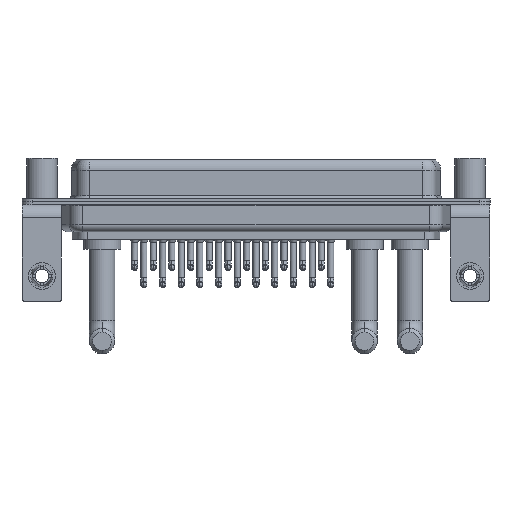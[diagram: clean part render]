
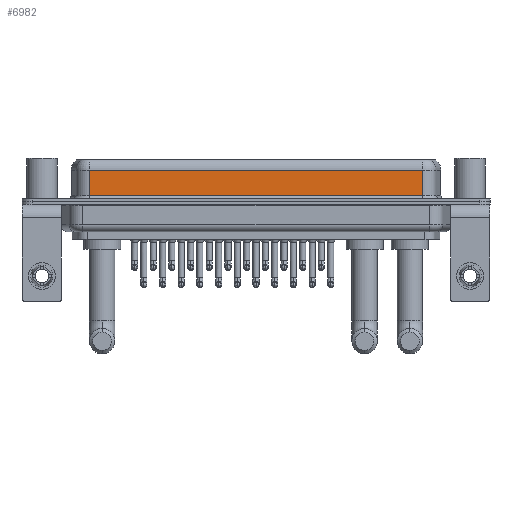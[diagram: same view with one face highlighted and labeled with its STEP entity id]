
A CAD part, front view. The second image highlights one B-rep face of the part: STEP entity #6982.
In plain terms, the highlighted planar face has unit normal (0, -1, 0).
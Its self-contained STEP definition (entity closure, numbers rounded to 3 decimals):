
#1175 = DIRECTION ( 'NONE',  ( 1., 0., 0. ) ) ;
#1801 = CARTESIAN_POINT ( 'NONE',  ( 56.462, -3.95, 6.4 ) ) ;
#2533 = ORIENTED_EDGE ( 'NONE', *, *, #26857, .T. ) ;
#2872 = VECTOR ( 'NONE', #3121, 1000. ) ;
#3121 = DIRECTION ( 'NONE',  ( -1., 0., 0. ) ) ;
#4502 = CARTESIAN_POINT ( 'NONE',  ( 7.038, -3.95, 4.65 ) ) ;
#6108 = DIRECTION ( 'NONE',  ( 0., 0., -1. ) ) ;
#6982 = ADVANCED_FACE ( 'NONE', ( #18783 ), #10620, .F. ) ;
#7758 = ORIENTED_EDGE ( 'NONE', *, *, #14734, .T. ) ;
#7822 = LINE ( 'NONE', #22518, #14104 ) ;
#8000 = CARTESIAN_POINT ( 'NONE',  ( 56.462, -3.95, 6.4 ) ) ;
#8579 = DIRECTION ( 'NONE',  ( 0., 0., -1. ) ) ;
#9319 = CARTESIAN_POINT ( 'NONE',  ( 7.038, -3.95, 0.9 ) ) ;
#9834 = EDGE_CURVE ( 'NONE', #12134, #17858, #7822, .T. ) ;
#10620 = PLANE ( 'NONE',  #21606 ) ;
#12134 = VERTEX_POINT ( 'NONE', #9319 ) ;
#12714 = ORIENTED_EDGE ( 'NONE', *, *, #9834, .T. ) ;
#13174 = CARTESIAN_POINT ( 'NONE',  ( 56.462, -3.95, 4.65 ) ) ;
#13313 = CARTESIAN_POINT ( 'NONE',  ( 56.462, -3.95, 0.9 ) ) ;
#13820 = ORIENTED_EDGE ( 'NONE', *, *, #13949, .F. ) ;
#13949 = EDGE_CURVE ( 'NONE', #15622, #17858, #20767, .T. ) ;
#14104 = VECTOR ( 'NONE', #1175, 1000. ) ;
#14351 = DIRECTION ( 'NONE',  ( 0., 1., 0. ) ) ;
#14560 = LINE ( 'NONE', #23147, #23358 ) ;
#14734 = EDGE_CURVE ( 'NONE', #15622, #16390, #22103, .T. ) ;
#15622 = VERTEX_POINT ( 'NONE', #13174 ) ;
#16007 = CARTESIAN_POINT ( 'NONE',  ( 56.462, -3.95, 4.65 ) ) ;
#16390 = VERTEX_POINT ( 'NONE', #4502 ) ;
#16580 = DIRECTION ( 'NONE',  ( 0., 0., 1. ) ) ;
#17858 = VERTEX_POINT ( 'NONE', #13313 ) ;
#18783 = FACE_OUTER_BOUND ( 'NONE', #21100, .T. ) ;
#20767 = LINE ( 'NONE', #1801, #22769 ) ;
#21100 = EDGE_LOOP ( 'NONE', ( #13820, #7758, #2533, #12714 ) ) ;
#21606 = AXIS2_PLACEMENT_3D ( 'NONE', #8000, #14351, #16580 ) ;
#22103 = LINE ( 'NONE', #16007, #2872 ) ;
#22518 = CARTESIAN_POINT ( 'NONE',  ( 56.462, -3.95, 0.9 ) ) ;
#22769 = VECTOR ( 'NONE', #8579, 1000. ) ;
#23147 = CARTESIAN_POINT ( 'NONE',  ( 7.038, -3.95, 6.4 ) ) ;
#23358 = VECTOR ( 'NONE', #6108, 1000. ) ;
#26857 = EDGE_CURVE ( 'NONE', #16390, #12134, #14560, .T. ) ;
